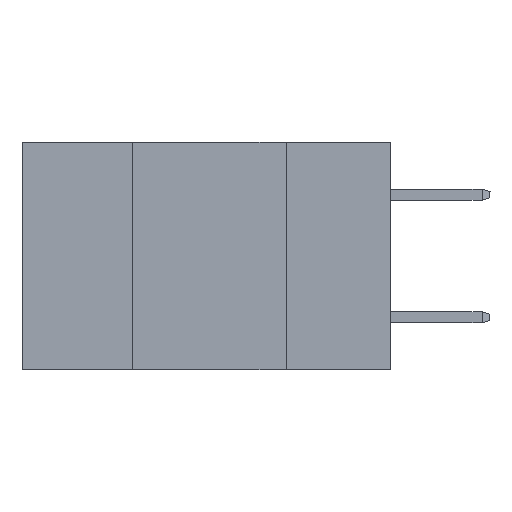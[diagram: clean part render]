
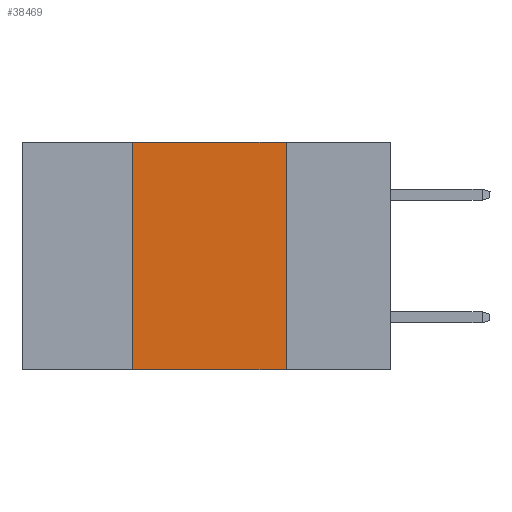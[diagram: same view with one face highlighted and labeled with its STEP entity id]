
A CAD part, left-side view. The second image highlights one B-rep face of the part: STEP entity #38469.
In plain terms, the highlighted planar face has unit normal (-1, 0, 0).
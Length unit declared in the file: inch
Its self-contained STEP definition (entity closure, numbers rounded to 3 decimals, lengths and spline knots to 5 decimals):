
#1085 = ORIENTED_EDGE ( 'NONE', *, *, #31122, .F. ) ;
#2030 = CARTESIAN_POINT ( 'NONE',  ( 0., 0.42, 0. ) ) ;
#2377 = EDGE_CURVE ( 'NONE', #26802, #28412, #35881, .T. ) ;
#4614 = LINE ( 'NONE', #36649, #19041 ) ;
#8909 = CARTESIAN_POINT ( 'NONE',  ( 0., 0.17, -0.37 ) ) ;
#12601 = ORIENTED_EDGE ( 'NONE', *, *, #20308, .F. ) ;
#13613 = VERTEX_POINT ( 'NONE', #2030 ) ;
#14764 = LINE ( 'NONE', #45116, #32002 ) ;
#15130 = AXIS2_PLACEMENT_3D ( 'NONE', #29706, #36894, #18830 ) ;
#15332 = DIRECTION ( 'NONE',  ( 0., -1., 0. ) ) ;
#18830 = DIRECTION ( 'NONE',  ( 0., 0., -1. ) ) ;
#19041 = VECTOR ( 'NONE', #15332, 39.37008 ) ;
#19559 = DIRECTION ( 'NONE',  ( 0., -1., 0. ) ) ;
#20308 = EDGE_CURVE ( 'NONE', #13613, #40732, #4614, .T. ) ;
#23179 = DIRECTION ( 'NONE',  ( 0., 0., -1. ) ) ;
#26405 = VECTOR ( 'NONE', #19559, 39.37008 ) ;
#26802 = VERTEX_POINT ( 'NONE', #37036 ) ;
#28267 = FACE_OUTER_BOUND ( 'NONE', #41444, .T. ) ;
#28412 = VERTEX_POINT ( 'NONE', #8909 ) ;
#29706 = CARTESIAN_POINT ( 'NONE',  ( 0., 0.6, 0. ) ) ;
#29838 = CARTESIAN_POINT ( 'NONE',  ( 0., 0.17, 0. ) ) ;
#29849 = PLANE ( 'NONE',  #15130 ) ;
#30925 = DIRECTION ( 'NONE',  ( 0., 0., 1. ) ) ;
#31122 = EDGE_CURVE ( 'NONE', #26802, #13613, #14764, .T. ) ;
#32002 = VECTOR ( 'NONE', #30925, 39.37008 ) ;
#33115 = EDGE_CURVE ( 'NONE', #40732, #28412, #45177, .T. ) ;
#35881 = LINE ( 'NONE', #44447, #26405 ) ;
#36649 = CARTESIAN_POINT ( 'NONE',  ( 0., 0.6, 0. ) ) ;
#36894 = DIRECTION ( 'NONE',  ( 1., 0., 0. ) ) ;
#37036 = CARTESIAN_POINT ( 'NONE',  ( 0., 0.42, -0.37 ) ) ;
#38469 = ADVANCED_FACE ( 'NONE', ( #28267 ), #29849, .F. ) ;
#40111 = ORIENTED_EDGE ( 'NONE', *, *, #2377, .T. ) ;
#40732 = VERTEX_POINT ( 'NONE', #29838 ) ;
#41444 = EDGE_LOOP ( 'NONE', ( #44910, #12601, #1085, #40111 ) ) ;
#44447 = CARTESIAN_POINT ( 'NONE',  ( 0., 0.6, -0.37 ) ) ;
#44495 = CARTESIAN_POINT ( 'NONE',  ( 0., 0.17, 0. ) ) ;
#44910 = ORIENTED_EDGE ( 'NONE', *, *, #33115, .F. ) ;
#45116 = CARTESIAN_POINT ( 'NONE',  ( 0., 0.42, 0. ) ) ;
#45177 = LINE ( 'NONE', #44495, #45756 ) ;
#45756 = VECTOR ( 'NONE', #23179, 39.37008 ) ;
